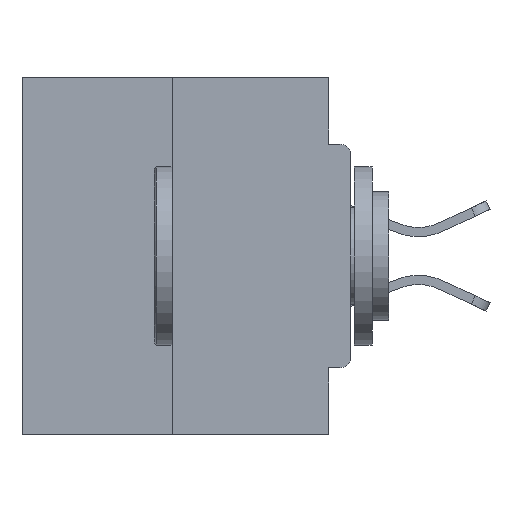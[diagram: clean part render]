
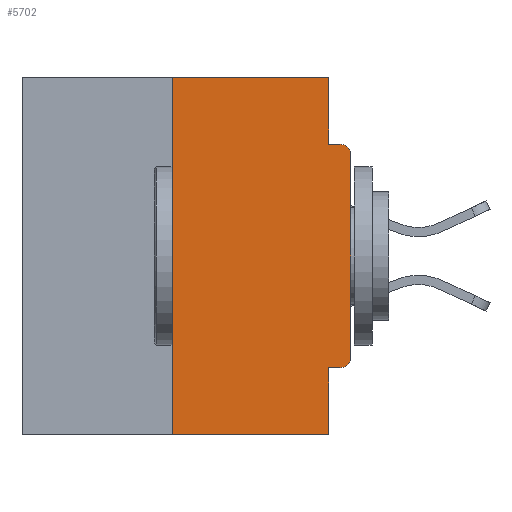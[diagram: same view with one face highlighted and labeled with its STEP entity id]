
A CAD part, left-side view. The second image highlights one B-rep face of the part: STEP entity #5702.
In plain terms, the highlighted planar face has unit normal (-1, 0, 0).
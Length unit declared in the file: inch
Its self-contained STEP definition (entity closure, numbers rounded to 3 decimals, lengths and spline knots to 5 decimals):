
#493 = LINE ( 'NONE', #1767, #17770 ) ;
#1074 = EDGE_CURVE ( 'NONE', #10916, #13538, #9468, .T. ) ;
#1217 = VERTEX_POINT ( 'NONE', #3803 ) ;
#1494 = DIRECTION ( 'NONE',  ( 0., 0., -1. ) ) ;
#1767 = CARTESIAN_POINT ( 'NONE',  ( 0., 0.031, -0.5 ) ) ;
#1983 = DIRECTION ( 'NONE',  ( 0., 0., -1. ) ) ;
#2158 = EDGE_CURVE ( 'NONE', #13538, #3852, #20321, .T. ) ;
#2217 = DIRECTION ( 'NONE',  ( 1., 0., 0. ) ) ;
#2673 = VECTOR ( 'NONE', #10298, 39.37008 ) ;
#2677 = CARTESIAN_POINT ( 'NONE',  ( 0., 0.46, 0. ) ) ;
#2906 = DIRECTION ( 'NONE',  ( 0., -1., 0. ) ) ;
#3142 = CARTESIAN_POINT ( 'NONE',  ( 0., 0., 0. ) ) ;
#3803 = CARTESIAN_POINT ( 'NONE',  ( 0., 0.25, 0. ) ) ;
#3852 = VERTEX_POINT ( 'NONE', #28275 ) ;
#4052 = DIRECTION ( 'NONE',  ( -1., 0., 0. ) ) ;
#4445 = CARTESIAN_POINT ( 'NONE',  ( 0., 0.015, -0.3915 ) ) ;
#5217 = CARTESIAN_POINT ( 'NONE',  ( 0., 0.46, 0. ) ) ;
#5607 = AXIS2_PLACEMENT_3D ( 'NONE', #5217, #2217, #1494 ) ;
#5702 = ADVANCED_FACE ( 'NONE', ( #23753 ), #22911, .F. ) ;
#6528 = DIRECTION ( 'NONE',  ( 0., 0., -1. ) ) ;
#8482 = VERTEX_POINT ( 'NONE', #24644 ) ;
#8875 = ORIENTED_EDGE ( 'NONE', *, *, #1074, .T. ) ;
#9468 = LINE ( 'NONE', #3142, #2673 ) ;
#9472 = DIRECTION ( 'NONE',  ( 0., 0., -1. ) ) ;
#9660 = EDGE_CURVE ( 'NONE', #15243, #8482, #31165, .T. ) ;
#9891 = ORIENTED_EDGE ( 'NONE', *, *, #25126, .F. ) ;
#10196 = EDGE_CURVE ( 'NONE', #15243, #1217, #17434, .T. ) ;
#10298 = DIRECTION ( 'NONE',  ( 0., 0., 1. ) ) ;
#10576 = VECTOR ( 'NONE', #13918, 39.37008 ) ;
#10916 = VERTEX_POINT ( 'NONE', #27432 ) ;
#10932 = VECTOR ( 'NONE', #2906, 39.37008 ) ;
#11257 = EDGE_CURVE ( 'NONE', #32623, #10916, #16648, .T. ) ;
#11326 = LINE ( 'NONE', #20682, #24236 ) ;
#11783 = CARTESIAN_POINT ( 'NONE',  ( 0., 0.031, 0. ) ) ;
#13538 = VERTEX_POINT ( 'NONE', #32685 ) ;
#13918 = DIRECTION ( 'NONE',  ( 0., 0., 1. ) ) ;
#14071 = CARTESIAN_POINT ( 'NONE',  ( 0., 0.031, -0.0935 ) ) ;
#14298 = EDGE_CURVE ( 'NONE', #19118, #3852, #11326, .T. ) ;
#14524 = ORIENTED_EDGE ( 'NONE', *, *, #14298, .F. ) ;
#14558 = CARTESIAN_POINT ( 'NONE',  ( 0., 0.46, -0.5 ) ) ;
#15100 = CARTESIAN_POINT ( 'NONE',  ( 0., 0., -0.4065 ) ) ;
#15243 = VERTEX_POINT ( 'NONE', #20204 ) ;
#16097 = VERTEX_POINT ( 'NONE', #27835 ) ;
#16648 = CIRCLE ( 'NONE', #33191, 0.015 ) ;
#16962 = AXIS2_PLACEMENT_3D ( 'NONE', #27349, #4052, #6528 ) ;
#17101 = EDGE_CURVE ( 'NONE', #1217, #16097, #31501, .T. ) ;
#17434 = LINE ( 'NONE', #29413, #10576 ) ;
#17770 = VECTOR ( 'NONE', #9472, 39.37008 ) ;
#18251 = EDGE_CURVE ( 'NONE', #23032, #8482, #493, .T. ) ;
#18330 = EDGE_CURVE ( 'NONE', #32623, #23032, #26639, .T. ) ;
#18602 = ORIENTED_EDGE ( 'NONE', *, *, #10196, .F. ) ;
#19118 = VERTEX_POINT ( 'NONE', #14071 ) ;
#19422 = VECTOR ( 'NONE', #22336, 39.37008 ) ;
#20184 = CARTESIAN_POINT ( 'NONE',  ( 0., 0.015, -0.4065 ) ) ;
#20204 = CARTESIAN_POINT ( 'NONE',  ( 0., 0.25, -0.5 ) ) ;
#20321 = CIRCLE ( 'NONE', #16962, 0.015 ) ;
#20682 = CARTESIAN_POINT ( 'NONE',  ( 0., 0., -0.0935 ) ) ;
#20783 = DIRECTION ( 'NONE',  ( 0., -1., 0. ) ) ;
#21795 = ORIENTED_EDGE ( 'NONE', *, *, #2158, .T. ) ;
#22336 = DIRECTION ( 'NONE',  ( 0., -1., 0. ) ) ;
#22911 = PLANE ( 'NONE',  #5607 ) ;
#23032 = VERTEX_POINT ( 'NONE', #28412 ) ;
#23753 = FACE_OUTER_BOUND ( 'NONE', #23801, .T. ) ;
#23801 = EDGE_LOOP ( 'NONE', ( #26476, #18602, #30319, #24595, #31623, #31999, #8875, #21795, #14524, #9891 ) ) ;
#24236 = VECTOR ( 'NONE', #20783, 39.37008 ) ;
#24595 = ORIENTED_EDGE ( 'NONE', *, *, #18251, .F. ) ;
#24644 = CARTESIAN_POINT ( 'NONE',  ( 0., 0.031, -0.5 ) ) ;
#24945 = DIRECTION ( 'NONE',  ( -1., 0., 0. ) ) ;
#25126 = EDGE_CURVE ( 'NONE', #16097, #19118, #28559, .T. ) ;
#26476 = ORIENTED_EDGE ( 'NONE', *, *, #17101, .F. ) ;
#26639 = LINE ( 'NONE', #15100, #27447 ) ;
#27349 = CARTESIAN_POINT ( 'NONE',  ( 0., 0.015, -0.1085 ) ) ;
#27356 = VECTOR ( 'NONE', #29618, 39.37008 ) ;
#27432 = CARTESIAN_POINT ( 'NONE',  ( 0., 0., -0.3915 ) ) ;
#27447 = VECTOR ( 'NONE', #33113, 39.37008 ) ;
#27835 = CARTESIAN_POINT ( 'NONE',  ( 0., 0.031, 0. ) ) ;
#28275 = CARTESIAN_POINT ( 'NONE',  ( 0., 0.015, -0.0935 ) ) ;
#28412 = CARTESIAN_POINT ( 'NONE',  ( 0., 0.031, -0.4065 ) ) ;
#28559 = LINE ( 'NONE', #11783, #27356 ) ;
#29413 = CARTESIAN_POINT ( 'NONE',  ( 0., 0.25, 0. ) ) ;
#29618 = DIRECTION ( 'NONE',  ( 0., 0., -1. ) ) ;
#30319 = ORIENTED_EDGE ( 'NONE', *, *, #9660, .T. ) ;
#31165 = LINE ( 'NONE', #14558, #19422 ) ;
#31501 = LINE ( 'NONE', #2677, #10932 ) ;
#31623 = ORIENTED_EDGE ( 'NONE', *, *, #18330, .F. ) ;
#31999 = ORIENTED_EDGE ( 'NONE', *, *, #11257, .T. ) ;
#32623 = VERTEX_POINT ( 'NONE', #20184 ) ;
#32685 = CARTESIAN_POINT ( 'NONE',  ( 0., 0., -0.1085 ) ) ;
#33113 = DIRECTION ( 'NONE',  ( 0., 1., 0. ) ) ;
#33191 = AXIS2_PLACEMENT_3D ( 'NONE', #4445, #24945, #1983 ) ;
